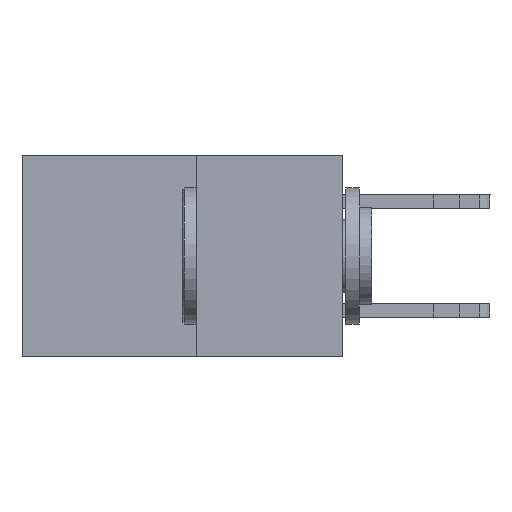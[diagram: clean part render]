
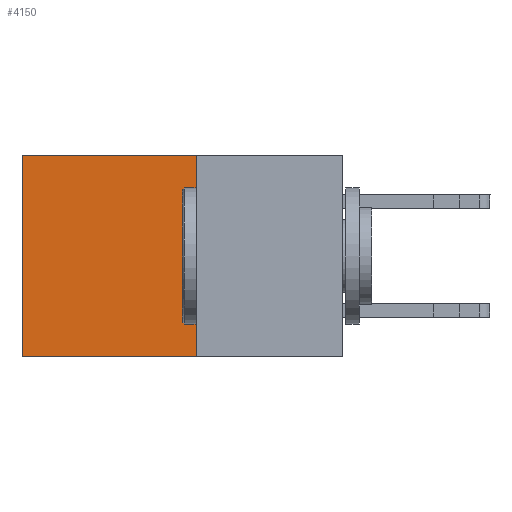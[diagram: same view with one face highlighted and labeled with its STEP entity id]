
A CAD part, left-side view. The second image highlights one B-rep face of the part: STEP entity #4150.
In plain terms, the highlighted planar face has unit normal (-1, 0, 0).
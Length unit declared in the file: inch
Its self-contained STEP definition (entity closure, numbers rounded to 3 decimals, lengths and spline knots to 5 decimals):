
#864 = ORIENTED_EDGE ( 'NONE', *, *, #15562, .T. ) ;
#1816 = LINE ( 'NONE', #2655, #10936 ) ;
#2655 = CARTESIAN_POINT ( 'NONE',  ( 0.277, 0.27, 0. ) ) ;
#2753 = DIRECTION ( 'NONE',  ( 0., 0., -1. ) ) ;
#3623 = ORIENTED_EDGE ( 'NONE', *, *, #12105, .T. ) ;
#4150 = ADVANCED_FACE ( 'NONE', ( #8576 ), #16278, .F. ) ;
#4437 = DIRECTION ( 'NONE',  ( 0., 0., -1. ) ) ;
#4941 = VERTEX_POINT ( 'NONE', #6743 ) ;
#6743 = CARTESIAN_POINT ( 'NONE',  ( 0.277, 0.27, 0. ) ) ;
#7005 = DIRECTION ( 'NONE',  ( 0., 0., -1. ) ) ;
#7788 = DIRECTION ( 'NONE',  ( 0., 1., 0. ) ) ;
#8184 = EDGE_CURVE ( 'NONE', #4941, #18915, #17684, .T. ) ;
#8284 = EDGE_LOOP ( 'NONE', ( #3623, #18925, #12805, #864 ) ) ;
#8410 = VERTEX_POINT ( 'NONE', #18080 ) ;
#8576 = FACE_OUTER_BOUND ( 'NONE', #8284, .T. ) ;
#8832 = LINE ( 'NONE', #17790, #10667 ) ;
#10667 = VECTOR ( 'NONE', #4437, 39.37008 ) ;
#10936 = VECTOR ( 'NONE', #7788, 39.37008 ) ;
#10950 = VECTOR ( 'NONE', #11814, 39.37008 ) ;
#10974 = CARTESIAN_POINT ( 'NONE',  ( 0.277, 0.27, -0.37 ) ) ;
#11144 = EDGE_CURVE ( 'NONE', #18915, #8410, #17762, .T. ) ;
#11814 = DIRECTION ( 'NONE',  ( 0., 1., 0. ) ) ;
#12105 = EDGE_CURVE ( 'NONE', #13117, #8410, #8832, .T. ) ;
#12805 = ORIENTED_EDGE ( 'NONE', *, *, #8184, .F. ) ;
#13117 = VERTEX_POINT ( 'NONE', #18704 ) ;
#14561 = CARTESIAN_POINT ( 'NONE',  ( 0.277, 0.27, -0.37 ) ) ;
#14667 = AXIS2_PLACEMENT_3D ( 'NONE', #16166, #18899, #7005 ) ;
#15562 = EDGE_CURVE ( 'NONE', #4941, #13117, #1816, .T. ) ;
#16118 = CARTESIAN_POINT ( 'NONE',  ( 0.277, 0.27, -0.37 ) ) ;
#16166 = CARTESIAN_POINT ( 'NONE',  ( 0.277, 0.27, -0.37 ) ) ;
#16278 = PLANE ( 'NONE',  #14667 ) ;
#16521 = VECTOR ( 'NONE', #2753, 39.37008 ) ;
#17684 = LINE ( 'NONE', #16118, #16521 ) ;
#17762 = LINE ( 'NONE', #14561, #10950 ) ;
#17790 = CARTESIAN_POINT ( 'NONE',  ( 0.277, 0.59, -0.37 ) ) ;
#18080 = CARTESIAN_POINT ( 'NONE',  ( 0.277, 0.59, -0.37 ) ) ;
#18704 = CARTESIAN_POINT ( 'NONE',  ( 0.277, 0.59, 0. ) ) ;
#18899 = DIRECTION ( 'NONE',  ( 1., 0., 0. ) ) ;
#18915 = VERTEX_POINT ( 'NONE', #10974 ) ;
#18925 = ORIENTED_EDGE ( 'NONE', *, *, #11144, .F. ) ;
